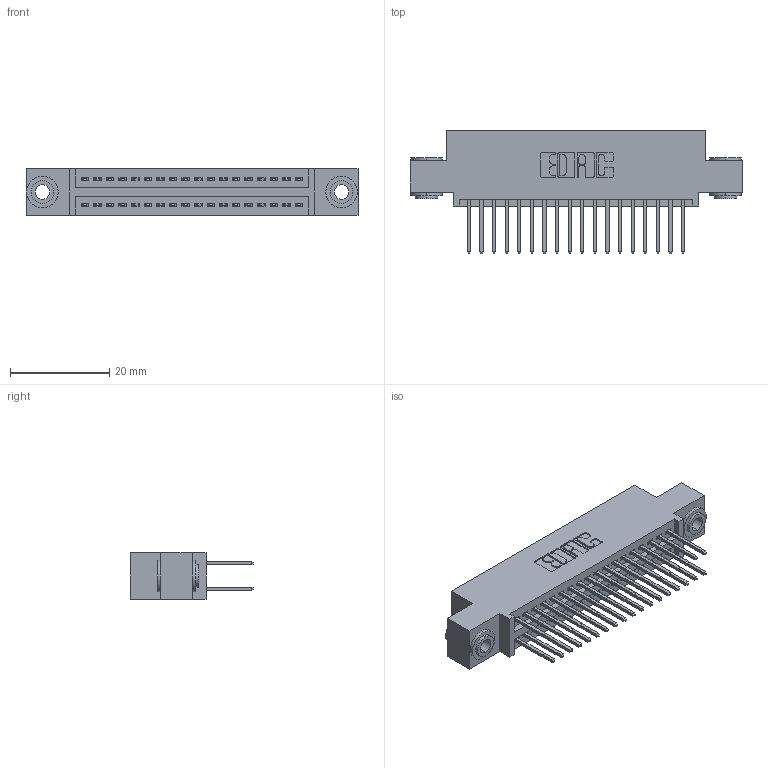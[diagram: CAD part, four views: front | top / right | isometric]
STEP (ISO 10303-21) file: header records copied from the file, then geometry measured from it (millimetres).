
FILE_DESCRIPTION (( 'STEP AP203' ), '1' );
FILE_NAME ('395-036-523-503.STEP', '2018-11-13T18:30:04', ( '' ), ( '' ), 'SwSTEP 2.0', 'SolidWorks 2016', '' );
FILE_SCHEMA (( 'CONFIG_CONTROL_DESIGN' ));
Length unit declared in the file: inch
Products named in the file (4): 345-250-002_345-250-002-102; 395-036-523-503; 345-292-001_345-293-123; 345 Part_0.110 Offset - 0.156 Dia-TH
Assembly tree (39 placements, depth 2):
  395-036-523-503
    345 Part_0.110 Offset - 0.156 Dia-TH
    345-292-001_345-293-123  x36
    345-250-002_345-250-002-102  x2
Bounding box: 66.93 x 24.82 x 9.4 mm (x, y, z)
Volume: 6298.6 mm3; surface area: 9474.3 mm2
Topology: 39 solids, 39 shells, 1968 faces, 5793 edges, 3810 vertices
Faces by surface type: plane 1282, cylinder 678, cone 8
Entity records: 18154 total; most frequent: CARTESIAN_POINT 3043, ORIENTED_EDGE 2970, DIRECTION 2743, EDGE_CURVE 1485, VECTOR 1257, LINE 1257, VERTEX_POINT 986, AXIS2_PLACEMENT_3D 743
